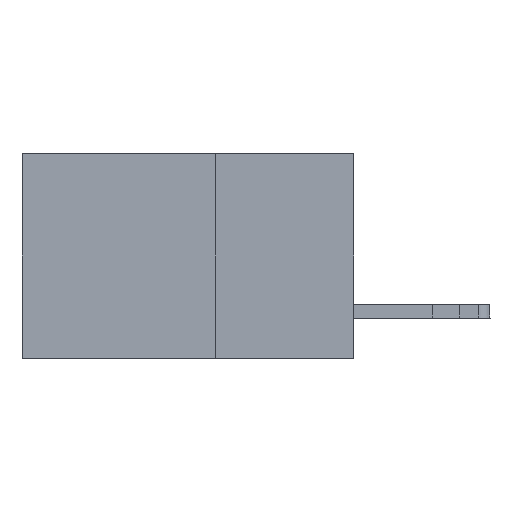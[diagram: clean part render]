
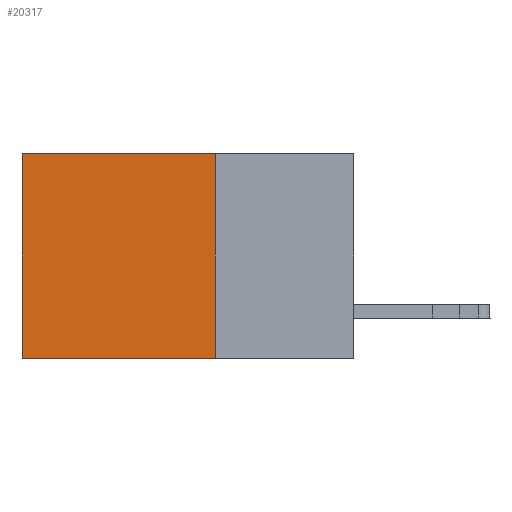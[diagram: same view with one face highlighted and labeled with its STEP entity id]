
A CAD part, left-side view. The second image highlights one B-rep face of the part: STEP entity #20317.
In plain terms, the highlighted planar face has unit normal (-1, 0, 0).
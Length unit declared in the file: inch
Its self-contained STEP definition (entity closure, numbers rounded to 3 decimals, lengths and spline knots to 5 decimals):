
#489 = VECTOR ( 'NONE', #3913, 39.37008 ) ;
#3190 = DIRECTION ( 'NONE',  ( 0., 0., -1. ) ) ;
#3913 = DIRECTION ( 'NONE',  ( 0., 1., 0. ) ) ;
#4580 = EDGE_CURVE ( 'NONE', #19293, #35352, #7784, .T. ) ;
#6595 = LINE ( 'NONE', #22407, #13686 ) ;
#7416 = DIRECTION ( 'NONE',  ( 0., 0., -1. ) ) ;
#7784 = LINE ( 'NONE', #35405, #21859 ) ;
#9072 = CARTESIAN_POINT ( 'NONE',  ( 0.2875, 0.25, -0.37 ) ) ;
#9198 = CARTESIAN_POINT ( 'NONE',  ( 0.2875, 0.25, 0. ) ) ;
#9605 = DIRECTION ( 'NONE',  ( 0., 1., 0. ) ) ;
#9641 = LINE ( 'NONE', #24516, #24618 ) ;
#9948 = EDGE_CURVE ( 'NONE', #35352, #19768, #32540, .T. ) ;
#11995 = ORIENTED_EDGE ( 'NONE', *, *, #9948, .F. ) ;
#13306 = ORIENTED_EDGE ( 'NONE', *, *, #37332, .T. ) ;
#13686 = VECTOR ( 'NONE', #7416, 39.37008 ) ;
#16803 = ORIENTED_EDGE ( 'NONE', *, *, #33436, .T. ) ;
#18229 = PLANE ( 'NONE',  #19678 ) ;
#19293 = VERTEX_POINT ( 'NONE', #21454 ) ;
#19678 = AXIS2_PLACEMENT_3D ( 'NONE', #9198, #21259, #3190 ) ;
#19768 = VERTEX_POINT ( 'NONE', #30292 ) ;
#20317 = ADVANCED_FACE ( 'NONE', ( #31055 ), #18229, .F. ) ;
#21259 = DIRECTION ( 'NONE',  ( 1., 0., 0. ) ) ;
#21454 = CARTESIAN_POINT ( 'NONE',  ( 0.2875, 0.25, 0. ) ) ;
#21859 = VECTOR ( 'NONE', #35531, 39.37008 ) ;
#22407 = CARTESIAN_POINT ( 'NONE',  ( 0.2875, 0.6, 0. ) ) ;
#23032 = EDGE_LOOP ( 'NONE', ( #16803, #11995, #38476, #13306 ) ) ;
#24516 = CARTESIAN_POINT ( 'NONE',  ( 0.2875, 0.25, 0. ) ) ;
#24618 = VECTOR ( 'NONE', #9605, 39.37008 ) ;
#30292 = CARTESIAN_POINT ( 'NONE',  ( 0.2875, 0.6, -0.37 ) ) ;
#30836 = CARTESIAN_POINT ( 'NONE',  ( 0.2875, 0.25, -0.37 ) ) ;
#31055 = FACE_OUTER_BOUND ( 'NONE', #23032, .T. ) ;
#32540 = LINE ( 'NONE', #30836, #489 ) ;
#33436 = EDGE_CURVE ( 'NONE', #33774, #19768, #6595, .T. ) ;
#33774 = VERTEX_POINT ( 'NONE', #35694 ) ;
#35352 = VERTEX_POINT ( 'NONE', #9072 ) ;
#35405 = CARTESIAN_POINT ( 'NONE',  ( 0.2875, 0.25, 0. ) ) ;
#35531 = DIRECTION ( 'NONE',  ( 0., 0., -1. ) ) ;
#35694 = CARTESIAN_POINT ( 'NONE',  ( 0.2875, 0.6, 0. ) ) ;
#37332 = EDGE_CURVE ( 'NONE', #19293, #33774, #9641, .T. ) ;
#38476 = ORIENTED_EDGE ( 'NONE', *, *, #4580, .F. ) ;
